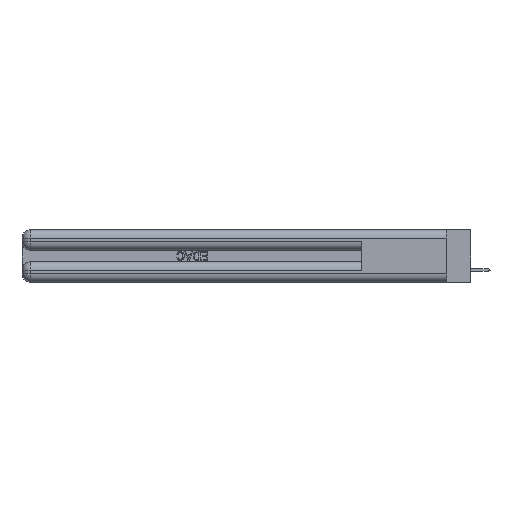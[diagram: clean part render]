
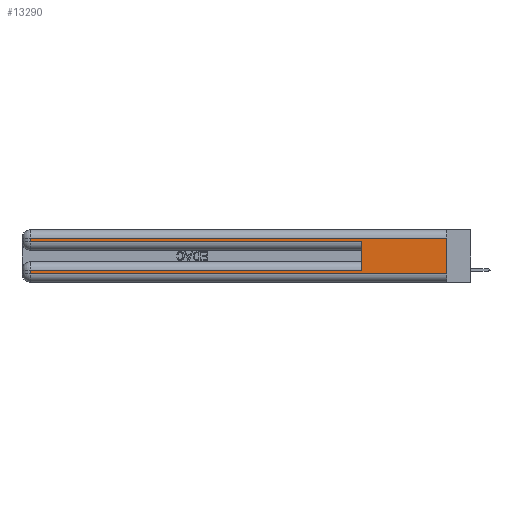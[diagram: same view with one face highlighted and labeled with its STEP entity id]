
A CAD part, left-side view. The second image highlights one B-rep face of the part: STEP entity #13290.
In plain terms, the highlighted planar face has unit normal (-1, 0, 0).
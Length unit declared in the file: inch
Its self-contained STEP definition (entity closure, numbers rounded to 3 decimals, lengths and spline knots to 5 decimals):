
#691 = DIRECTION ( 'NONE',  ( 0., 0., 1. ) ) ;
#906 = CARTESIAN_POINT ( 'NONE',  ( 0., 0., 0.085 ) ) ;
#1569 = EDGE_CURVE ( 'NONE', #5904, #24490, #16153, .T. ) ;
#4680 = CARTESIAN_POINT ( 'NONE',  ( 0., 2.94, 0.31 ) ) ;
#5389 = DIRECTION ( 'NONE',  ( 0., 0., -1. ) ) ;
#5611 = CARTESIAN_POINT ( 'NONE',  ( 0., 0., 0.31 ) ) ;
#5879 = ORIENTED_EDGE ( 'NONE', *, *, #16278, .T. ) ;
#5904 = VERTEX_POINT ( 'NONE', #7067 ) ;
#6285 = EDGE_CURVE ( 'NONE', #40315, #14536, #23874, .T. ) ;
#6945 = VECTOR ( 'NONE', #31508, 39.37008 ) ;
#7067 = CARTESIAN_POINT ( 'NONE',  ( 0., 0.6, 0.085 ) ) ;
#7090 = VECTOR ( 'NONE', #691, 39.37008 ) ;
#7466 = DIRECTION ( 'NONE',  ( 0., -1., 0. ) ) ;
#8298 = EDGE_CURVE ( 'NONE', #11311, #40315, #48467, .T. ) ;
#8666 = CARTESIAN_POINT ( 'NONE',  ( 0., 2.94, 0.285 ) ) ;
#8874 = ORIENTED_EDGE ( 'NONE', *, *, #27559, .T. ) ;
#10716 = PLANE ( 'NONE',  #20943 ) ;
#11311 = VERTEX_POINT ( 'NONE', #5611 ) ;
#13290 = ADVANCED_FACE ( 'NONE', ( #23028 ), #10716, .F. ) ;
#14410 = DIRECTION ( 'NONE',  ( 0., 0., -1. ) ) ;
#14536 = VERTEX_POINT ( 'NONE', #8666 ) ;
#15388 = DIRECTION ( 'NONE',  ( 0., 1., 0. ) ) ;
#16153 = LINE ( 'NONE', #906, #35456 ) ;
#16278 = EDGE_CURVE ( 'NONE', #25285, #37328, #48309, .T. ) ;
#16447 = CARTESIAN_POINT ( 'NONE',  ( 0., 2.94, 0.37 ) ) ;
#16533 = CARTESIAN_POINT ( 'NONE',  ( 0., 0., 0.37 ) ) ;
#17002 = ORIENTED_EDGE ( 'NONE', *, *, #1569, .T. ) ;
#17242 = ORIENTED_EDGE ( 'NONE', *, *, #20287, .F. ) ;
#18128 = EDGE_CURVE ( 'NONE', #11311, #37328, #38996, .T. ) ;
#19334 = CARTESIAN_POINT ( 'NONE',  ( 0., 2.94, 0.06 ) ) ;
#19815 = ORIENTED_EDGE ( 'NONE', *, *, #8298, .T. ) ;
#20222 = ORIENTED_EDGE ( 'NONE', *, *, #6285, .T. ) ;
#20287 = EDGE_CURVE ( 'NONE', #5904, #21953, #46785, .T. ) ;
#20943 = AXIS2_PLACEMENT_3D ( 'NONE', #48708, #38083, #14410 ) ;
#21953 = VERTEX_POINT ( 'NONE', #31166 ) ;
#23028 = FACE_OUTER_BOUND ( 'NONE', #32909, .T. ) ;
#23142 = CARTESIAN_POINT ( 'NONE',  ( 0., 2.94, 0.085 ) ) ;
#23874 = LINE ( 'NONE', #31271, #26337 ) ;
#24490 = VERTEX_POINT ( 'NONE', #23142 ) ;
#25285 = VERTEX_POINT ( 'NONE', #19334 ) ;
#25722 = VECTOR ( 'NONE', #36711, 39.37008 ) ;
#26173 = ORIENTED_EDGE ( 'NONE', *, *, #18128, .F. ) ;
#26208 = LINE ( 'NONE', #40519, #40527 ) ;
#26337 = VECTOR ( 'NONE', #5389, 39.37008 ) ;
#27559 = EDGE_CURVE ( 'NONE', #14536, #21953, #26208, .T. ) ;
#31166 = CARTESIAN_POINT ( 'NONE',  ( 0., 0.6, 0.285 ) ) ;
#31271 = CARTESIAN_POINT ( 'NONE',  ( 0., 2.94, 0.37 ) ) ;
#31456 = DIRECTION ( 'NONE',  ( 0., 1., 0. ) ) ;
#31508 = DIRECTION ( 'NONE',  ( 0., 0., -1. ) ) ;
#32909 = EDGE_LOOP ( 'NONE', ( #26173, #19815, #20222, #8874, #17242, #17002, #45223, #5879 ) ) ;
#35382 = CARTESIAN_POINT ( 'NONE',  ( 0., 0., 0.06 ) ) ;
#35456 = VECTOR ( 'NONE', #31456, 39.37008 ) ;
#36427 = LINE ( 'NONE', #16447, #6945 ) ;
#36711 = DIRECTION ( 'NONE',  ( 0., -1., 0. ) ) ;
#37328 = VERTEX_POINT ( 'NONE', #35382 ) ;
#38083 = DIRECTION ( 'NONE',  ( 1., 0., 0. ) ) ;
#38996 = LINE ( 'NONE', #16533, #41633 ) ;
#39675 = CARTESIAN_POINT ( 'NONE',  ( 0., 0., 0.06 ) ) ;
#40315 = VERTEX_POINT ( 'NONE', #4680 ) ;
#40519 = CARTESIAN_POINT ( 'NONE',  ( 0., 0., 0.285 ) ) ;
#40527 = VECTOR ( 'NONE', #7466, 39.37008 ) ;
#41633 = VECTOR ( 'NONE', #43191, 39.37008 ) ;
#42096 = VECTOR ( 'NONE', #15388, 39.37008 ) ;
#43191 = DIRECTION ( 'NONE',  ( 0., 0., -1. ) ) ;
#45223 = ORIENTED_EDGE ( 'NONE', *, *, #46380, .T. ) ;
#45250 = CARTESIAN_POINT ( 'NONE',  ( 0., 0., 0.31 ) ) ;
#46300 = CARTESIAN_POINT ( 'NONE',  ( 0., 0.6, 0.145 ) ) ;
#46380 = EDGE_CURVE ( 'NONE', #24490, #25285, #36427, .T. ) ;
#46785 = LINE ( 'NONE', #46300, #7090 ) ;
#48309 = LINE ( 'NONE', #39675, #25722 ) ;
#48467 = LINE ( 'NONE', #45250, #42096 ) ;
#48708 = CARTESIAN_POINT ( 'NONE',  ( 0., 0., 0.37 ) ) ;
